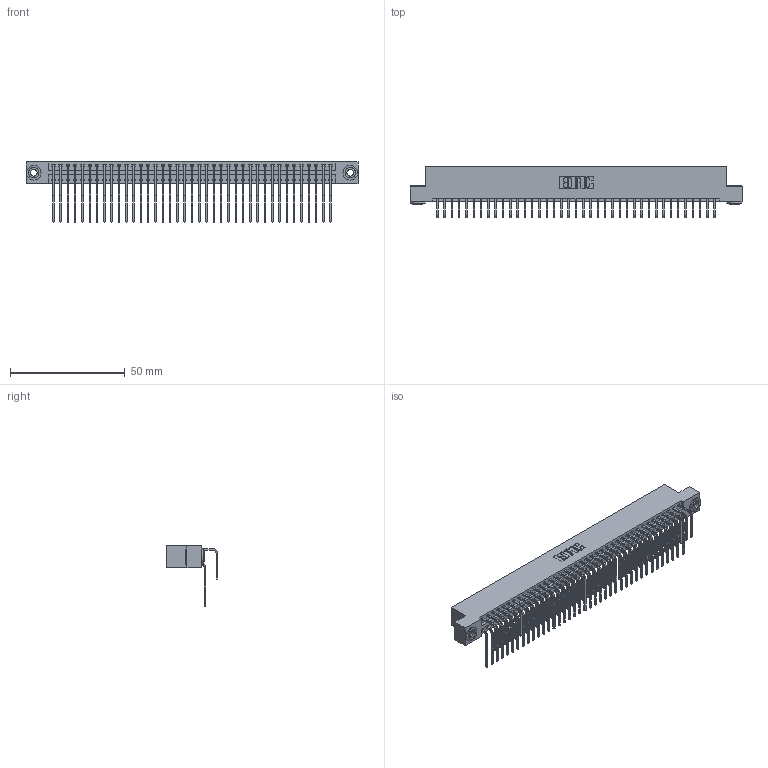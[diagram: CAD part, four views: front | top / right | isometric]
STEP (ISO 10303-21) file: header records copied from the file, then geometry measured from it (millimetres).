
FILE_DESCRIPTION (( 'STEP AP203' ), '1' );
FILE_NAME ('346-078-558-203.STEP', '2022-05-25T14:38:06', ( '' ), ( '' ), 'SwSTEP 2.0', 'SolidWorks 2020', '' );
FILE_SCHEMA (( 'CONFIG_CONTROL_DESIGN' ));
Length unit declared in the file: inch
Products named in the file (5): 346 Part_Flush Mounting Lugs - 0.156 Dia-TH; 345-250-002_345-250-002-102; 346-078-558-203; 345-292-001_558 559 Tail - 1; 345-292-001_558 Tail - 2
Assembly tree (81 placements, depth 2):
  346-078-558-203
    346 Part_Flush Mounting Lugs - 0.156 Dia-TH
    345-292-001_558 559 Tail - 1  x39
    345-292-001_558 Tail - 2  x39
    345-250-002_345-250-002-102  x2
Bounding box: 144.4 x 22.16 x 26.16 mm (x, y, z)
Volume: 14508.7 mm3; surface area: 22303.3 mm2
Topology: 81 solids, 81 shells, 4386 faces, 12999 edges, 8558 vertices
Faces by surface type: plane 2986, cylinder 1392, cone 8
Entity records: 28706 total; most frequent: CARTESIAN_POINT 4768, ORIENTED_EDGE 4642, DIRECTION 4255, EDGE_CURVE 2321, VECTOR 1969, LINE 1969, VERTEX_POINT 1542, AXIS2_PLACEMENT_3D 1143
